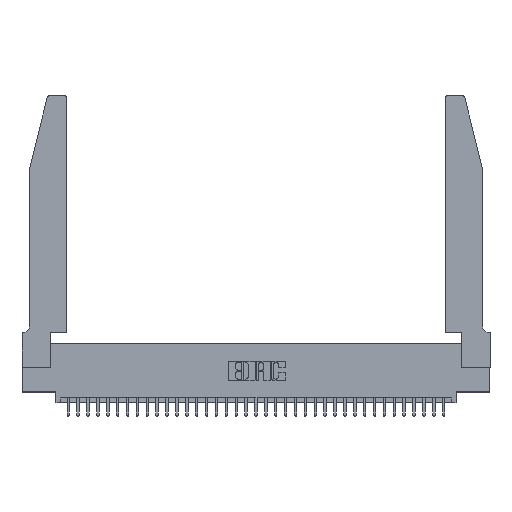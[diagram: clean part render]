
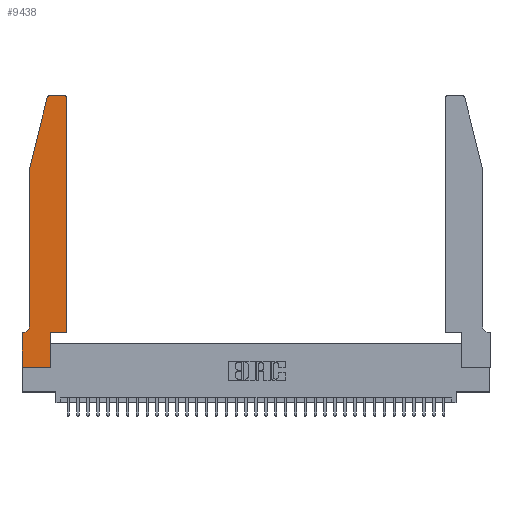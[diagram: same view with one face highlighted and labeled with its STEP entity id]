
A CAD part, top view. The second image highlights one B-rep face of the part: STEP entity #9438.
In plain terms, the highlighted planar face has unit normal (0, 0, 1).
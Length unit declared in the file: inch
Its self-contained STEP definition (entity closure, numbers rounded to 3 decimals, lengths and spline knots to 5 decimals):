
#351 = DIRECTION ( 'NONE',  ( 0., 0., 1. ) ) ;
#718 = DIRECTION ( 'NONE',  ( 0., -1., 0. ) ) ;
#887 = CARTESIAN_POINT ( 'NONE',  ( 0.2605, 2.75, 0.37 ) ) ;
#1978 = ORIENTED_EDGE ( 'NONE', *, *, #27342, .T. ) ;
#2283 = VERTEX_POINT ( 'NONE', #32861 ) ;
#2328 = DIRECTION ( 'NONE',  ( 0., 0., 1. ) ) ;
#2505 = CARTESIAN_POINT ( 'NONE',  ( 0.4205, 2.75, 0.37 ) ) ;
#3578 = ORIENTED_EDGE ( 'NONE', *, *, #17382, .T. ) ;
#3928 = EDGE_LOOP ( 'NONE', ( #29814, #22929, #15258, #1978, #8885, #22935, #3996, #6601, #33592, #18003, #14846, #3578 ) ) ;
#3996 = ORIENTED_EDGE ( 'NONE', *, *, #11901, .T. ) ;
#4224 = AXIS2_PLACEMENT_3D ( 'NONE', #21031, #4462, #23834 ) ;
#4462 = DIRECTION ( 'NONE',  ( 0., 0., 1. ) ) ;
#4701 = DIRECTION ( 'NONE',  ( 0., 1., 0. ) ) ;
#4923 = EDGE_CURVE ( 'NONE', #30586, #27868, #26215, .T. ) ;
#4951 = CARTESIAN_POINT ( 'NONE',  ( 0.2865, 0.35, 0.37 ) ) ;
#5221 = VERTEX_POINT ( 'NONE', #9647 ) ;
#5429 = AXIS2_PLACEMENT_3D ( 'NONE', #33401, #33070, #27574 ) ;
#6601 = ORIENTED_EDGE ( 'NONE', *, *, #16509, .T. ) ;
#6831 = CARTESIAN_POINT ( 'NONE',  ( 0., 0., 0.37 ) ) ;
#6882 = EDGE_CURVE ( 'NONE', #28488, #8531, #29132, .T. ) ;
#7134 = CARTESIAN_POINT ( 'NONE',  ( 0.25487, 2.72718, 0.37 ) ) ;
#7270 = DIRECTION ( 'NONE',  ( 0., -1., 0. ) ) ;
#8531 = VERTEX_POINT ( 'NONE', #13388 ) ;
#8885 = ORIENTED_EDGE ( 'NONE', *, *, #6882, .T. ) ;
#9438 = ADVANCED_FACE ( 'NONE', ( #27243 ), #16878, .T. ) ;
#9647 = CARTESIAN_POINT ( 'NONE',  ( 0., 0.35, 0.37 ) ) ;
#9972 = CARTESIAN_POINT ( 'NONE',  ( 0.4505, 0.35, 0.37 ) ) ;
#10047 = DIRECTION ( 'NONE',  ( -1., 0., 0. ) ) ;
#10164 = CARTESIAN_POINT ( 'NONE',  ( 0.4505, 0.35, 0.37 ) ) ;
#11901 = EDGE_CURVE ( 'NONE', #5221, #2283, #31041, .T. ) ;
#12612 = VERTEX_POINT ( 'NONE', #12738 ) ;
#12738 = CARTESIAN_POINT ( 'NONE',  ( 0.284, 2.75, 0.37 ) ) ;
#12870 = DIRECTION ( 'NONE',  ( 0., 1., 0. ) ) ;
#13277 = VECTOR ( 'NONE', #12870, 39.37008 ) ;
#13346 = VECTOR ( 'NONE', #7270, 39.37008 ) ;
#13388 = CARTESIAN_POINT ( 'NONE',  ( 0.0055, 0.35, 0.37 ) ) ;
#14846 = ORIENTED_EDGE ( 'NONE', *, *, #28446, .T. ) ;
#14933 = EDGE_CURVE ( 'NONE', #8531, #5221, #23547, .T. ) ;
#15037 = LINE ( 'NONE', #16664, #17162 ) ;
#15258 = ORIENTED_EDGE ( 'NONE', *, *, #35454, .T. ) ;
#15539 = VERTEX_POINT ( 'NONE', #7134 ) ;
#15652 = VERTEX_POINT ( 'NONE', #25800 ) ;
#16441 = DIRECTION ( 'NONE',  ( 1., 0., 0. ) ) ;
#16509 = EDGE_CURVE ( 'NONE', #2283, #30586, #29018, .T. ) ;
#16556 = LINE ( 'NONE', #887, #23467 ) ;
#16664 = CARTESIAN_POINT ( 'NONE',  ( 0.0755, 2., 0.37 ) ) ;
#16878 = PLANE ( 'NONE',  #35178 ) ;
#16979 = CARTESIAN_POINT ( 'NONE',  ( 0., 0.35, 0.37 ) ) ;
#17145 = EDGE_CURVE ( 'NONE', #12612, #15539, #21219, .T. ) ;
#17162 = VECTOR ( 'NONE', #19329, 39.37008 ) ;
#17382 = EDGE_CURVE ( 'NONE', #28656, #19959, #28929, .T. ) ;
#18003 = ORIENTED_EDGE ( 'NONE', *, *, #34614, .T. ) ;
#18266 = DIRECTION ( 'NONE',  ( 1., 0., 0. ) ) ;
#19329 = DIRECTION ( 'NONE',  ( -0.239, -0.971, 0. ) ) ;
#19959 = VERTEX_POINT ( 'NONE', #2505 ) ;
#20030 = DIRECTION ( 'NONE',  ( -1., 0., 0. ) ) ;
#20650 = VECTOR ( 'NONE', #718, 39.37008 ) ;
#21031 = CARTESIAN_POINT ( 'NONE',  ( 0.284, 2.72, 0.37 ) ) ;
#21219 = CIRCLE ( 'NONE', #4224, 0.03 ) ;
#21302 = CARTESIAN_POINT ( 'NONE',  ( 0.2865, 0., 0.37 ) ) ;
#21726 = VECTOR ( 'NONE', #16441, 39.37008 ) ;
#22651 = VECTOR ( 'NONE', #10047, 39.37008 ) ;
#22657 = CARTESIAN_POINT ( 'NONE',  ( 0.0755, 2., 0.37 ) ) ;
#22929 = ORIENTED_EDGE ( 'NONE', *, *, #17145, .T. ) ;
#22935 = ORIENTED_EDGE ( 'NONE', *, *, #14933, .T. ) ;
#23467 = VECTOR ( 'NONE', #20030, 39.37008 ) ;
#23547 = LINE ( 'NONE', #28615, #22651 ) ;
#23834 = DIRECTION ( 'NONE',  ( 1., 0., 0. ) ) ;
#24729 = CARTESIAN_POINT ( 'NONE',  ( 0.4505, 2.72, 0.37 ) ) ;
#25309 = DIRECTION ( 'NONE',  ( 1., 0., 0. ) ) ;
#25800 = CARTESIAN_POINT ( 'NONE',  ( 0.0755, 2., 0.37 ) ) ;
#26215 = LINE ( 'NONE', #34849, #30998 ) ;
#26591 = VERTEX_POINT ( 'NONE', #31891 ) ;
#27243 = FACE_OUTER_BOUND ( 'NONE', #3928, .T. ) ;
#27342 = EDGE_CURVE ( 'NONE', #15652, #28488, #31066, .T. ) ;
#27574 = DIRECTION ( 'NONE',  ( -1., 0., 0. ) ) ;
#27629 = LINE ( 'NONE', #10164, #28020 ) ;
#27868 = VERTEX_POINT ( 'NONE', #4951 ) ;
#28020 = VECTOR ( 'NONE', #18266, 39.37008 ) ;
#28446 = EDGE_CURVE ( 'NONE', #26591, #28656, #32761, .T. ) ;
#28488 = VERTEX_POINT ( 'NONE', #34682 ) ;
#28615 = CARTESIAN_POINT ( 'NONE',  ( 0.0755, 0.35, 0.37 ) ) ;
#28656 = VERTEX_POINT ( 'NONE', #24729 ) ;
#28929 = CIRCLE ( 'NONE', #28996, 0.03 ) ;
#28996 = AXIS2_PLACEMENT_3D ( 'NONE', #35296, #2328, #29663 ) ;
#29018 = LINE ( 'NONE', #6831, #21726 ) ;
#29132 = CIRCLE ( 'NONE', #5429, 0.07 ) ;
#29663 = DIRECTION ( 'NONE',  ( 1., 0., 0. ) ) ;
#29814 = ORIENTED_EDGE ( 'NONE', *, *, #32552, .T. ) ;
#30586 = VERTEX_POINT ( 'NONE', #21302 ) ;
#30998 = VECTOR ( 'NONE', #4701, 39.37008 ) ;
#31041 = LINE ( 'NONE', #31329, #13346 ) ;
#31066 = LINE ( 'NONE', #22657, #20650 ) ;
#31329 = CARTESIAN_POINT ( 'NONE',  ( 0., 0., 0.37 ) ) ;
#31891 = CARTESIAN_POINT ( 'NONE',  ( 0.4505, 0.35, 0.37 ) ) ;
#32552 = EDGE_CURVE ( 'NONE', #19959, #12612, #16556, .T. ) ;
#32761 = LINE ( 'NONE', #9972, #13277 ) ;
#32861 = CARTESIAN_POINT ( 'NONE',  ( 0., 0., 0.37 ) ) ;
#33070 = DIRECTION ( 'NONE',  ( 0., 0., -1. ) ) ;
#33401 = CARTESIAN_POINT ( 'NONE',  ( 0.0055, 0.42, 0.37 ) ) ;
#33592 = ORIENTED_EDGE ( 'NONE', *, *, #4923, .T. ) ;
#34614 = EDGE_CURVE ( 'NONE', #27868, #26591, #27629, .T. ) ;
#34682 = CARTESIAN_POINT ( 'NONE',  ( 0.0755, 0.42, 0.37 ) ) ;
#34849 = CARTESIAN_POINT ( 'NONE',  ( 0.2865, 0.35, 0.37 ) ) ;
#35178 = AXIS2_PLACEMENT_3D ( 'NONE', #16979, #351, #25309 ) ;
#35296 = CARTESIAN_POINT ( 'NONE',  ( 0.4205, 2.72, 0.37 ) ) ;
#35454 = EDGE_CURVE ( 'NONE', #15539, #15652, #15037, .T. ) ;
